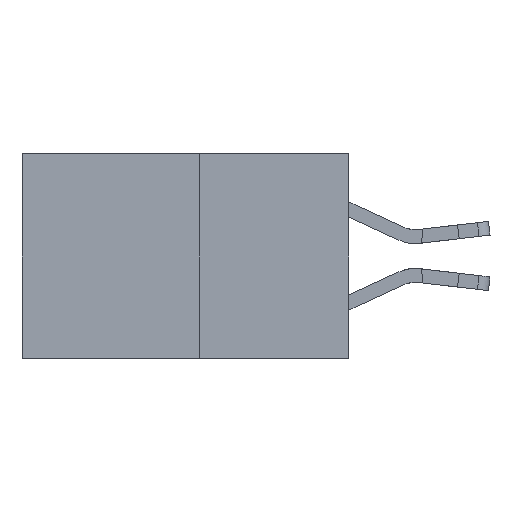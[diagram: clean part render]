
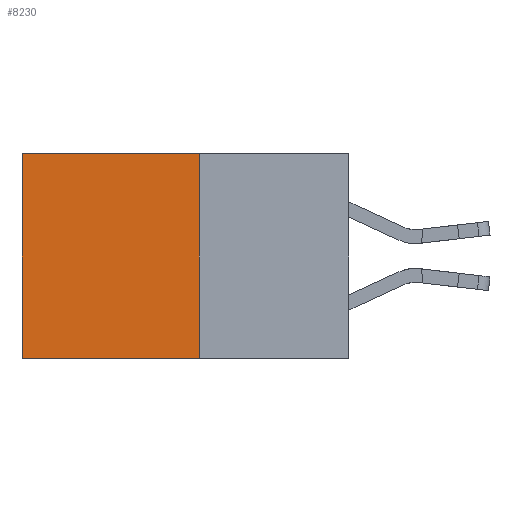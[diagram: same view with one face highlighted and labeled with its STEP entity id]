
A CAD part, left-side view. The second image highlights one B-rep face of the part: STEP entity #8230.
In plain terms, the highlighted planar face has unit normal (-1, 0, 0).
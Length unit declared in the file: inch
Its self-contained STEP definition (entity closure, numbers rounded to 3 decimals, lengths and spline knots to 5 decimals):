
#209 = CARTESIAN_POINT ( 'NONE',  ( 0.277, 0.27, -0.37 ) ) ;
#258 = PLANE ( 'NONE',  #18838 ) ;
#1220 = VERTEX_POINT ( 'NONE', #4714 ) ;
#1238 = CARTESIAN_POINT ( 'NONE',  ( 0.277, 0.27, -0.37 ) ) ;
#1639 = ORIENTED_EDGE ( 'NONE', *, *, #13427, .T. ) ;
#2705 = CARTESIAN_POINT ( 'NONE',  ( 0.277, 0.27, 0. ) ) ;
#4133 = ORIENTED_EDGE ( 'NONE', *, *, #19850, .F. ) ;
#4714 = CARTESIAN_POINT ( 'NONE',  ( 0.277, 0.59, -0.37 ) ) ;
#4739 = DIRECTION ( 'NONE',  ( 1., 0., 0. ) ) ;
#4852 = VERTEX_POINT ( 'NONE', #20290 ) ;
#5444 = FACE_OUTER_BOUND ( 'NONE', #14008, .T. ) ;
#5528 = LINE ( 'NONE', #15292, #18331 ) ;
#5758 = DIRECTION ( 'NONE',  ( 0., 0., -1. ) ) ;
#5771 = ORIENTED_EDGE ( 'NONE', *, *, #15217, .T. ) ;
#7189 = LINE ( 'NONE', #10831, #11618 ) ;
#8098 = VERTEX_POINT ( 'NONE', #1238 ) ;
#8230 = ADVANCED_FACE ( 'NONE', ( #5444 ), #258, .F. ) ;
#9700 = LINE ( 'NONE', #2705, #14103 ) ;
#9776 = DIRECTION ( 'NONE',  ( 0., 1., 0. ) ) ;
#9820 = CARTESIAN_POINT ( 'NONE',  ( 0.277, 0.59, 0. ) ) ;
#10831 = CARTESIAN_POINT ( 'NONE',  ( 0.277, 0.27, -0.37 ) ) ;
#11618 = VECTOR ( 'NONE', #5758, 39.37008 ) ;
#12385 = EDGE_CURVE ( 'NONE', #4852, #8098, #7189, .T. ) ;
#12770 = DIRECTION ( 'NONE',  ( 0., 1., 0. ) ) ;
#13427 = EDGE_CURVE ( 'NONE', #18482, #1220, #5528, .T. ) ;
#14008 = EDGE_LOOP ( 'NONE', ( #1639, #4133, #16284, #5771 ) ) ;
#14103 = VECTOR ( 'NONE', #12770, 39.37008 ) ;
#14825 = VECTOR ( 'NONE', #9776, 39.37008 ) ;
#15217 = EDGE_CURVE ( 'NONE', #4852, #18482, #9700, .T. ) ;
#15292 = CARTESIAN_POINT ( 'NONE',  ( 0.277, 0.59, -0.37 ) ) ;
#16284 = ORIENTED_EDGE ( 'NONE', *, *, #12385, .F. ) ;
#16433 = DIRECTION ( 'NONE',  ( 0., 0., -1. ) ) ;
#16973 = DIRECTION ( 'NONE',  ( 0., 0., -1. ) ) ;
#18331 = VECTOR ( 'NONE', #16973, 39.37008 ) ;
#18482 = VERTEX_POINT ( 'NONE', #9820 ) ;
#18838 = AXIS2_PLACEMENT_3D ( 'NONE', #209, #4739, #16433 ) ;
#19241 = LINE ( 'NONE', #19694, #14825 ) ;
#19694 = CARTESIAN_POINT ( 'NONE',  ( 0.277, 0.27, -0.37 ) ) ;
#19850 = EDGE_CURVE ( 'NONE', #8098, #1220, #19241, .T. ) ;
#20290 = CARTESIAN_POINT ( 'NONE',  ( 0.277, 0.27, 0. ) ) ;
